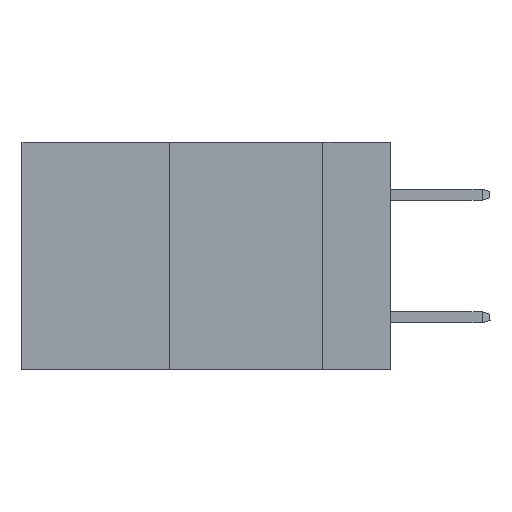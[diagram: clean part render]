
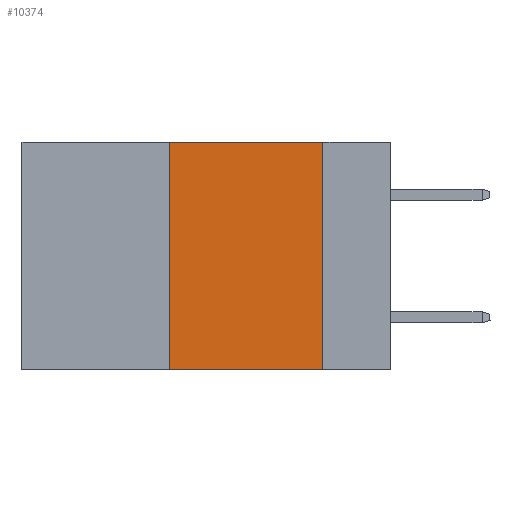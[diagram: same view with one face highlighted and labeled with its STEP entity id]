
A CAD part, left-side view. The second image highlights one B-rep face of the part: STEP entity #10374.
In plain terms, the highlighted planar face has unit normal (-1, 0, 0).
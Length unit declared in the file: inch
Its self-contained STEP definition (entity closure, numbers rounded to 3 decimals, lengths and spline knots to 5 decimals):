
#1071 = CARTESIAN_POINT ( 'NONE',  ( 0., 0.36, 0. ) ) ;
#1933 = CARTESIAN_POINT ( 'NONE',  ( 0., 0.11, 0. ) ) ;
#3799 = LINE ( 'NONE', #14174, #18369 ) ;
#5719 = CARTESIAN_POINT ( 'NONE',  ( 0., 0.6, 0. ) ) ;
#6370 = LINE ( 'NONE', #1933, #14838 ) ;
#8407 = DIRECTION ( 'NONE',  ( 0., -1., 0. ) ) ;
#9182 = VERTEX_POINT ( 'NONE', #22744 ) ;
#9589 = LINE ( 'NONE', #27628, #11044 ) ;
#10374 = ADVANCED_FACE ( 'NONE', ( #18972 ), #13714, .F. ) ;
#11044 = VECTOR ( 'NONE', #17557, 39.37008 ) ;
#11464 = CARTESIAN_POINT ( 'NONE',  ( 0., 0.36, -0.37 ) ) ;
#13668 = EDGE_CURVE ( 'NONE', #33167, #26590, #9589, .T. ) ;
#13714 = PLANE ( 'NONE',  #27209 ) ;
#13732 = ORIENTED_EDGE ( 'NONE', *, *, #28402, .F. ) ;
#14174 = CARTESIAN_POINT ( 'NONE',  ( 0., 0.6, 0. ) ) ;
#14838 = VECTOR ( 'NONE', #22189, 39.37008 ) ;
#15518 = ORIENTED_EDGE ( 'NONE', *, *, #13668, .T. ) ;
#16846 = ORIENTED_EDGE ( 'NONE', *, *, #28840, .F. ) ;
#17557 = DIRECTION ( 'NONE',  ( 0., -1., 0. ) ) ;
#18369 = VECTOR ( 'NONE', #8407, 39.37008 ) ;
#18972 = FACE_OUTER_BOUND ( 'NONE', #31194, .T. ) ;
#19724 = VERTEX_POINT ( 'NONE', #23293 ) ;
#20427 = EDGE_CURVE ( 'NONE', #19724, #9182, #3799, .T. ) ;
#21869 = DIRECTION ( 'NONE',  ( 0., 0., -1. ) ) ;
#22189 = DIRECTION ( 'NONE',  ( 0., 0., -1. ) ) ;
#22475 = DIRECTION ( 'NONE',  ( 0., 0., 1. ) ) ;
#22744 = CARTESIAN_POINT ( 'NONE',  ( 0., 0.11, 0. ) ) ;
#23293 = CARTESIAN_POINT ( 'NONE',  ( 0., 0.36, 0. ) ) ;
#24347 = CARTESIAN_POINT ( 'NONE',  ( 0., 0.11, -0.37 ) ) ;
#24875 = LINE ( 'NONE', #1071, #31191 ) ;
#26590 = VERTEX_POINT ( 'NONE', #24347 ) ;
#27209 = AXIS2_PLACEMENT_3D ( 'NONE', #5719, #31931, #21869 ) ;
#27628 = CARTESIAN_POINT ( 'NONE',  ( 0., 0.6, -0.37 ) ) ;
#27956 = ORIENTED_EDGE ( 'NONE', *, *, #20427, .F. ) ;
#28402 = EDGE_CURVE ( 'NONE', #9182, #26590, #6370, .T. ) ;
#28840 = EDGE_CURVE ( 'NONE', #33167, #19724, #24875, .T. ) ;
#31191 = VECTOR ( 'NONE', #22475, 39.37008 ) ;
#31194 = EDGE_LOOP ( 'NONE', ( #13732, #27956, #16846, #15518 ) ) ;
#31931 = DIRECTION ( 'NONE',  ( 1., 0., 0. ) ) ;
#33167 = VERTEX_POINT ( 'NONE', #11464 ) ;
